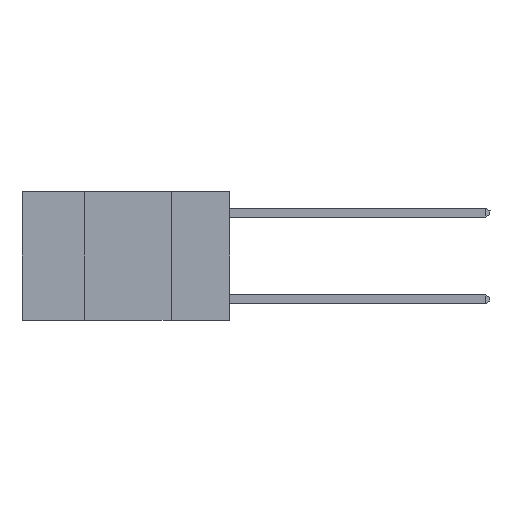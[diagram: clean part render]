
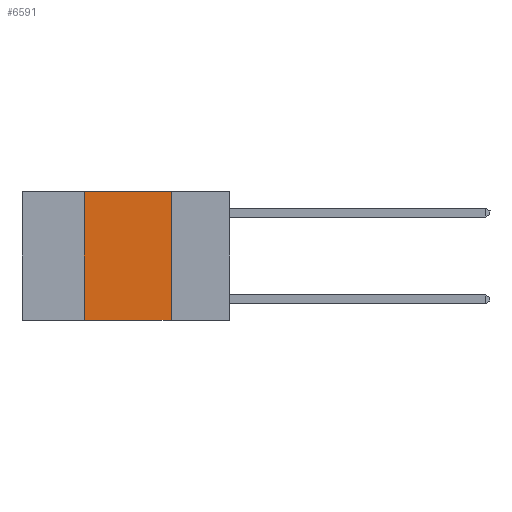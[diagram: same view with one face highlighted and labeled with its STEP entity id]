
A CAD part, left-side view. The second image highlights one B-rep face of the part: STEP entity #6591.
In plain terms, the highlighted planar face has unit normal (-1, 0, 0).
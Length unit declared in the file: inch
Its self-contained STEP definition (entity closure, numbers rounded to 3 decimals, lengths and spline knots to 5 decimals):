
#86 = DIRECTION ( 'NONE',  ( 1., 0., 0. ) ) ;
#185 = VERTEX_POINT ( 'NONE', #8937 ) ;
#432 = CARTESIAN_POINT ( 'NONE',  ( 0., 0.17, -0.37 ) ) ;
#1034 = EDGE_CURVE ( 'NONE', #185, #16181, #5411, .T. ) ;
#2061 = CARTESIAN_POINT ( 'NONE',  ( 0., 0.6, 0. ) ) ;
#3555 = FACE_OUTER_BOUND ( 'NONE', #16019, .T. ) ;
#5411 = LINE ( 'NONE', #10155, #10206 ) ;
#6569 = EDGE_CURVE ( 'NONE', #15349, #16181, #17641, .T. ) ;
#6591 = ADVANCED_FACE ( 'NONE', ( #3555 ), #18170, .F. ) ;
#7629 = DIRECTION ( 'NONE',  ( 0., -1., 0. ) ) ;
#8051 = VECTOR ( 'NONE', #18151, 39.37008 ) ;
#8088 = ORIENTED_EDGE ( 'NONE', *, *, #15325, .F. ) ;
#8096 = DIRECTION ( 'NONE',  ( 0., 0., 1. ) ) ;
#8308 = LINE ( 'NONE', #2061, #8051 ) ;
#8528 = DIRECTION ( 'NONE',  ( 0., 0., -1. ) ) ;
#8937 = CARTESIAN_POINT ( 'NONE',  ( 0., 0.17, 0. ) ) ;
#9596 = CARTESIAN_POINT ( 'NONE',  ( 0., 0.6, -0.37 ) ) ;
#10109 = CARTESIAN_POINT ( 'NONE',  ( 0., 0.6, 0. ) ) ;
#10155 = CARTESIAN_POINT ( 'NONE',  ( 0., 0.17, 0. ) ) ;
#10206 = VECTOR ( 'NONE', #15160, 39.37008 ) ;
#10207 = AXIS2_PLACEMENT_3D ( 'NONE', #10109, #86, #8528 ) ;
#10255 = ORIENTED_EDGE ( 'NONE', *, *, #6569, .T. ) ;
#10852 = CARTESIAN_POINT ( 'NONE',  ( 0., 0.42, 0. ) ) ;
#11442 = LINE ( 'NONE', #19098, #14065 ) ;
#14065 = VECTOR ( 'NONE', #8096, 39.37008 ) ;
#15135 = EDGE_CURVE ( 'NONE', #15349, #18113, #11442, .T. ) ;
#15160 = DIRECTION ( 'NONE',  ( 0., 0., -1. ) ) ;
#15325 = EDGE_CURVE ( 'NONE', #18113, #185, #8308, .T. ) ;
#15349 = VERTEX_POINT ( 'NONE', #18567 ) ;
#15383 = ORIENTED_EDGE ( 'NONE', *, *, #15135, .F. ) ;
#16019 = EDGE_LOOP ( 'NONE', ( #16067, #8088, #15383, #10255 ) ) ;
#16067 = ORIENTED_EDGE ( 'NONE', *, *, #1034, .F. ) ;
#16181 = VERTEX_POINT ( 'NONE', #432 ) ;
#17641 = LINE ( 'NONE', #9596, #18239 ) ;
#18113 = VERTEX_POINT ( 'NONE', #10852 ) ;
#18151 = DIRECTION ( 'NONE',  ( 0., -1., 0. ) ) ;
#18170 = PLANE ( 'NONE',  #10207 ) ;
#18239 = VECTOR ( 'NONE', #7629, 39.37008 ) ;
#18567 = CARTESIAN_POINT ( 'NONE',  ( 0., 0.42, -0.37 ) ) ;
#19098 = CARTESIAN_POINT ( 'NONE',  ( 0., 0.42, 0. ) ) ;
